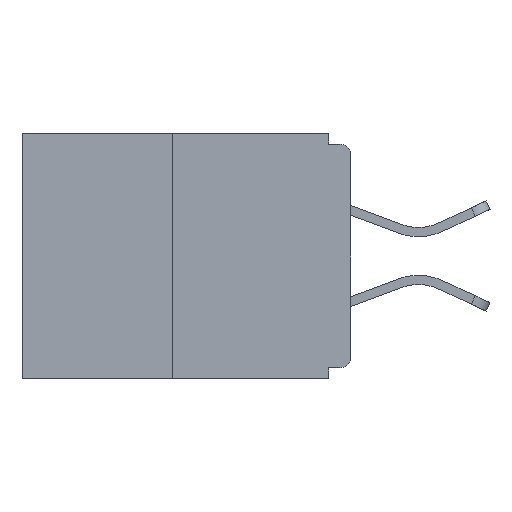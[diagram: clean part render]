
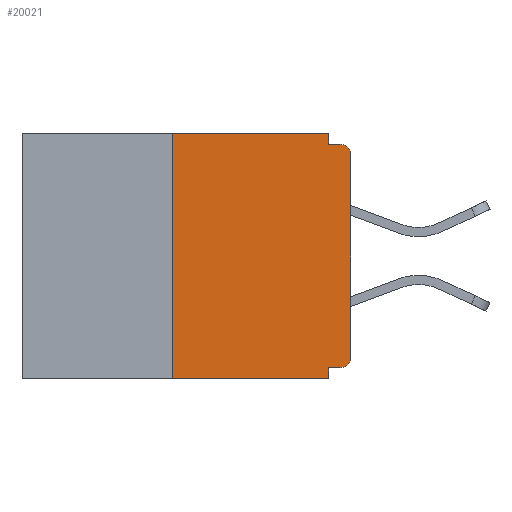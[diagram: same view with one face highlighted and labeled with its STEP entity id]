
A CAD part, left-side view. The second image highlights one B-rep face of the part: STEP entity #20021.
In plain terms, the highlighted planar face has unit normal (-1, 0, 0).
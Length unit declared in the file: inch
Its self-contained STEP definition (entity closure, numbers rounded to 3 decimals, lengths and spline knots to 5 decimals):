
#498 = CIRCLE ( 'NONE', #30214, 0.015 ) ;
#1351 = LINE ( 'NONE', #5115, #27203 ) ;
#1755 = LINE ( 'NONE', #6362, #25621 ) ;
#1771 = VERTEX_POINT ( 'NONE', #10434 ) ;
#1778 = CARTESIAN_POINT ( 'NONE',  ( 0., 0.46, -0.343 ) ) ;
#2279 = CARTESIAN_POINT ( 'NONE',  ( 0., 0.031, -0.015 ) ) ;
#3052 = ORIENTED_EDGE ( 'NONE', *, *, #11048, .T. ) ;
#3980 = CARTESIAN_POINT ( 'NONE',  ( 0., 0.031, 0. ) ) ;
#4020 = VERTEX_POINT ( 'NONE', #21622 ) ;
#4234 = PLANE ( 'NONE',  #27017 ) ;
#4427 = ORIENTED_EDGE ( 'NONE', *, *, #30526, .F. ) ;
#4805 = AXIS2_PLACEMENT_3D ( 'NONE', #19692, #9535, #9645 ) ;
#5115 = CARTESIAN_POINT ( 'NONE',  ( 0., 0., 0. ) ) ;
#5540 = EDGE_CURVE ( 'NONE', #26069, #15063, #17872, .T. ) ;
#6056 = DIRECTION ( 'NONE',  ( 0., 1., 0. ) ) ;
#6362 = CARTESIAN_POINT ( 'NONE',  ( 0., 0.031, -0.343 ) ) ;
#6604 = EDGE_CURVE ( 'NONE', #1771, #13089, #1755, .T. ) ;
#6752 = CARTESIAN_POINT ( 'NONE',  ( 0., 0.46, 0. ) ) ;
#7263 = EDGE_CURVE ( 'NONE', #7465, #1771, #21684, .T. ) ;
#7271 = DIRECTION ( 'NONE',  ( 0., 0., -1. ) ) ;
#7465 = VERTEX_POINT ( 'NONE', #19245 ) ;
#7536 = ORIENTED_EDGE ( 'NONE', *, *, #7263, .F. ) ;
#7788 = CARTESIAN_POINT ( 'NONE',  ( 0., 0.46, 0. ) ) ;
#8242 = EDGE_CURVE ( 'NONE', #21126, #13089, #30263, .T. ) ;
#9202 = DIRECTION ( 'NONE',  ( 0., 0., -1. ) ) ;
#9535 = DIRECTION ( 'NONE',  ( -1., 0., 0. ) ) ;
#9645 = DIRECTION ( 'NONE',  ( 0., 0., -1. ) ) ;
#10434 = CARTESIAN_POINT ( 'NONE',  ( 0., 0.031, -0.328 ) ) ;
#11048 = EDGE_CURVE ( 'NONE', #14815, #27376, #31263, .T. ) ;
#11637 = VERTEX_POINT ( 'NONE', #23975 ) ;
#11670 = DIRECTION ( 'NONE',  ( 0., 0., 1. ) ) ;
#11714 = CARTESIAN_POINT ( 'NONE',  ( 0., 0.015, -0.313 ) ) ;
#11858 = VECTOR ( 'NONE', #19678, 39.37008 ) ;
#11919 = DIRECTION ( 'NONE',  ( 0., 0., -1. ) ) ;
#12581 = FACE_OUTER_BOUND ( 'NONE', #23694, .T. ) ;
#13089 = VERTEX_POINT ( 'NONE', #23586 ) ;
#13235 = EDGE_CURVE ( 'NONE', #21126, #4020, #30683, .T. ) ;
#14646 = ORIENTED_EDGE ( 'NONE', *, *, #8242, .T. ) ;
#14709 = CARTESIAN_POINT ( 'NONE',  ( 0., 0.25, -0.343 ) ) ;
#14815 = VERTEX_POINT ( 'NONE', #20902 ) ;
#15063 = VERTEX_POINT ( 'NONE', #2279 ) ;
#15767 = VECTOR ( 'NONE', #11670, 39.37008 ) ;
#16300 = ORIENTED_EDGE ( 'NONE', *, *, #32468, .F. ) ;
#17149 = DIRECTION ( 'NONE',  ( 0., 0., -1. ) ) ;
#17581 = CARTESIAN_POINT ( 'NONE',  ( 0., 0., -0.015 ) ) ;
#17766 = CARTESIAN_POINT ( 'NONE',  ( 0., 0.031, 0. ) ) ;
#17821 = DIRECTION ( 'NONE',  ( 0., 0., 1. ) ) ;
#17872 = LINE ( 'NONE', #3980, #30792 ) ;
#18483 = LINE ( 'NONE', #17581, #11858 ) ;
#18598 = ORIENTED_EDGE ( 'NONE', *, *, #18812, .T. ) ;
#18635 = CARTESIAN_POINT ( 'NONE',  ( 0., 0.015, -0.015 ) ) ;
#18812 = EDGE_CURVE ( 'NONE', #11637, #14815, #1351, .T. ) ;
#19245 = CARTESIAN_POINT ( 'NONE',  ( 0., 0.015, -0.328 ) ) ;
#19678 = DIRECTION ( 'NONE',  ( 0., -1., 0. ) ) ;
#19692 = CARTESIAN_POINT ( 'NONE',  ( 0., 0.015, -0.03 ) ) ;
#19777 = DIRECTION ( 'NONE',  ( -1., 0., 0. ) ) ;
#20021 = ADVANCED_FACE ( 'NONE', ( #12581 ), #4234, .F. ) ;
#20413 = DIRECTION ( 'NONE',  ( 0., -1., 0. ) ) ;
#20520 = VECTOR ( 'NONE', #20413, 39.37008 ) ;
#20902 = CARTESIAN_POINT ( 'NONE',  ( 0., 0., -0.03 ) ) ;
#21126 = VERTEX_POINT ( 'NONE', #14709 ) ;
#21622 = CARTESIAN_POINT ( 'NONE',  ( 0., 0.25, 0. ) ) ;
#21684 = LINE ( 'NONE', #23235, #25196 ) ;
#22489 = ORIENTED_EDGE ( 'NONE', *, *, #32184, .T. ) ;
#23235 = CARTESIAN_POINT ( 'NONE',  ( 0., 0., -0.328 ) ) ;
#23586 = CARTESIAN_POINT ( 'NONE',  ( 0., 0.031, -0.343 ) ) ;
#23694 = EDGE_LOOP ( 'NONE', ( #4427, #31614, #14646, #29080, #7536, #22489, #18598, #3052, #16300, #30512 ) ) ;
#23975 = CARTESIAN_POINT ( 'NONE',  ( 0., 0., -0.313 ) ) ;
#24234 = DIRECTION ( 'NONE',  ( 0., -1., 0. ) ) ;
#24287 = DIRECTION ( 'NONE',  ( 1., 0., 0. ) ) ;
#24807 = VECTOR ( 'NONE', #24234, 39.37008 ) ;
#25196 = VECTOR ( 'NONE', #6056, 39.37008 ) ;
#25621 = VECTOR ( 'NONE', #9202, 39.37008 ) ;
#26069 = VERTEX_POINT ( 'NONE', #17766 ) ;
#27017 = AXIS2_PLACEMENT_3D ( 'NONE', #6752, #24287, #11919 ) ;
#27203 = VECTOR ( 'NONE', #17821, 39.37008 ) ;
#27376 = VERTEX_POINT ( 'NONE', #18635 ) ;
#29080 = ORIENTED_EDGE ( 'NONE', *, *, #6604, .F. ) ;
#30214 = AXIS2_PLACEMENT_3D ( 'NONE', #11714, #19777, #17149 ) ;
#30263 = LINE ( 'NONE', #1778, #24807 ) ;
#30512 = ORIENTED_EDGE ( 'NONE', *, *, #5540, .F. ) ;
#30526 = EDGE_CURVE ( 'NONE', #4020, #26069, #31908, .T. ) ;
#30683 = LINE ( 'NONE', #31903, #15767 ) ;
#30792 = VECTOR ( 'NONE', #7271, 39.37008 ) ;
#31263 = CIRCLE ( 'NONE', #4805, 0.015 ) ;
#31614 = ORIENTED_EDGE ( 'NONE', *, *, #13235, .F. ) ;
#31903 = CARTESIAN_POINT ( 'NONE',  ( 0., 0.25, 0. ) ) ;
#31908 = LINE ( 'NONE', #7788, #20520 ) ;
#32184 = EDGE_CURVE ( 'NONE', #7465, #11637, #498, .T. ) ;
#32468 = EDGE_CURVE ( 'NONE', #15063, #27376, #18483, .T. ) ;
